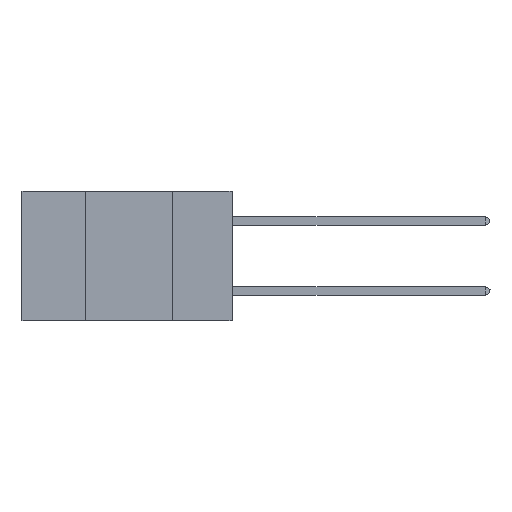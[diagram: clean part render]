
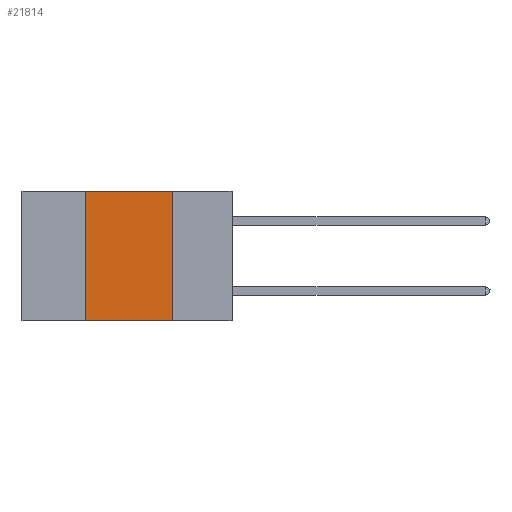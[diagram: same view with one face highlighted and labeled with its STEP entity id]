
A CAD part, left-side view. The second image highlights one B-rep face of the part: STEP entity #21814.
In plain terms, the highlighted planar face has unit normal (-1, 0, 0).
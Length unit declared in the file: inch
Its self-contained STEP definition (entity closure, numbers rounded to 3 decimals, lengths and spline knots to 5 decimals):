
#74 = CARTESIAN_POINT ( 'NONE',  ( 0., 0.6, 0. ) ) ;
#184 = CARTESIAN_POINT ( 'NONE',  ( 0., 0.17, 0. ) ) ;
#2688 = ORIENTED_EDGE ( 'NONE', *, *, #13355, .F. ) ;
#2705 = VERTEX_POINT ( 'NONE', #22441 ) ;
#5071 = LINE ( 'NONE', #74, #22708 ) ;
#5108 = LINE ( 'NONE', #13601, #6798 ) ;
#6656 = LINE ( 'NONE', #184, #12040 ) ;
#6715 = LINE ( 'NONE', #13594, #17083 ) ;
#6798 = VECTOR ( 'NONE', #26963, 39.37008 ) ;
#7248 = CARTESIAN_POINT ( 'NONE',  ( 0., 0.42, -0.37 ) ) ;
#7545 = CARTESIAN_POINT ( 'NONE',  ( 0., 0.42, 0. ) ) ;
#10550 = PLANE ( 'NONE',  #11912 ) ;
#10976 = DIRECTION ( 'NONE',  ( 1., 0., 0. ) ) ;
#11240 = DIRECTION ( 'NONE',  ( 0., -1., 0. ) ) ;
#11912 = AXIS2_PLACEMENT_3D ( 'NONE', #15229, #10976, #28466 ) ;
#12040 = VECTOR ( 'NONE', #25099, 39.37008 ) ;
#13355 = EDGE_CURVE ( 'NONE', #27366, #2705, #5071, .T. ) ;
#13594 = CARTESIAN_POINT ( 'NONE',  ( 0., 0.6, -0.37 ) ) ;
#13601 = CARTESIAN_POINT ( 'NONE',  ( 0., 0.42, 0. ) ) ;
#14688 = ORIENTED_EDGE ( 'NONE', *, *, #25012, .F. ) ;
#15229 = CARTESIAN_POINT ( 'NONE',  ( 0., 0.6, 0. ) ) ;
#15292 = ORIENTED_EDGE ( 'NONE', *, *, #22891, .F. ) ;
#17083 = VECTOR ( 'NONE', #11240, 39.37008 ) ;
#19477 = FACE_OUTER_BOUND ( 'NONE', #25943, .T. ) ;
#19735 = VERTEX_POINT ( 'NONE', #7248 ) ;
#21814 = ADVANCED_FACE ( 'NONE', ( #19477 ), #10550, .F. ) ;
#21819 = ORIENTED_EDGE ( 'NONE', *, *, #22394, .T. ) ;
#22394 = EDGE_CURVE ( 'NONE', #19735, #25462, #6715, .T. ) ;
#22441 = CARTESIAN_POINT ( 'NONE',  ( 0., 0.17, 0. ) ) ;
#22493 = DIRECTION ( 'NONE',  ( 0., -1., 0. ) ) ;
#22708 = VECTOR ( 'NONE', #22493, 39.37008 ) ;
#22891 = EDGE_CURVE ( 'NONE', #19735, #27366, #5108, .T. ) ;
#25012 = EDGE_CURVE ( 'NONE', #2705, #25462, #6656, .T. ) ;
#25099 = DIRECTION ( 'NONE',  ( 0., 0., -1. ) ) ;
#25462 = VERTEX_POINT ( 'NONE', #26845 ) ;
#25943 = EDGE_LOOP ( 'NONE', ( #14688, #2688, #15292, #21819 ) ) ;
#26845 = CARTESIAN_POINT ( 'NONE',  ( 0., 0.17, -0.37 ) ) ;
#26963 = DIRECTION ( 'NONE',  ( 0., 0., 1. ) ) ;
#27366 = VERTEX_POINT ( 'NONE', #7545 ) ;
#28466 = DIRECTION ( 'NONE',  ( 0., 0., -1. ) ) ;
